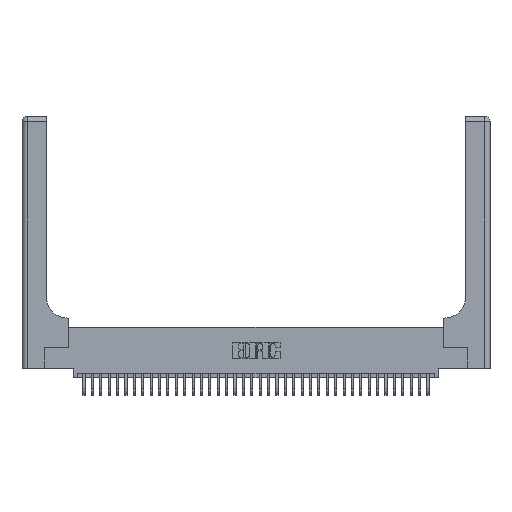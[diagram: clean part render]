
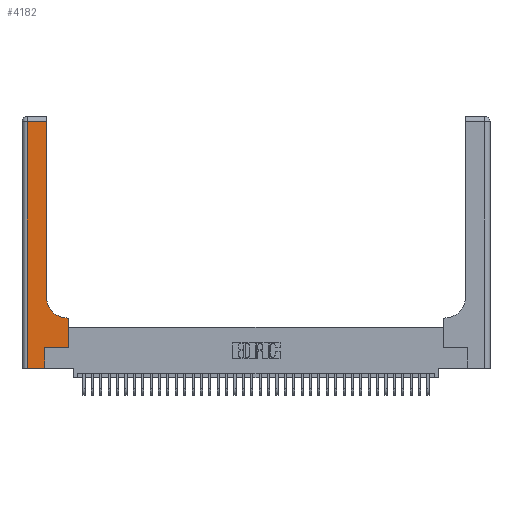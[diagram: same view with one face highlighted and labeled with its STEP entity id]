
A CAD part, top view. The second image highlights one B-rep face of the part: STEP entity #4182.
In plain terms, the highlighted planar face has unit normal (0, 0, 1).
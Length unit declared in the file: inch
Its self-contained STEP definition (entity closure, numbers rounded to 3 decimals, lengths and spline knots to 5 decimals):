
#35 = EDGE_CURVE ( 'NONE', #37936, #5996, #28060, .T. ) ;
#514 = CARTESIAN_POINT ( 'NONE',  ( 0., 0., 0.37 ) ) ;
#1296 = EDGE_CURVE ( 'NONE', #23925, #3361, #37200, .T. ) ;
#1332 = ORIENTED_EDGE ( 'NONE', *, *, #4130, .T. ) ;
#1995 = VECTOR ( 'NONE', #19127, 39.37008 ) ;
#2058 = EDGE_CURVE ( 'NONE', #7646, #23925, #10102, .T. ) ;
#2326 = FACE_OUTER_BOUND ( 'NONE', #29178, .T. ) ;
#3023 = DIRECTION ( 'NONE',  ( 0., 1., 0. ) ) ;
#3274 = LINE ( 'NONE', #15315, #38043 ) ;
#3361 = VERTEX_POINT ( 'NONE', #17592 ) ;
#4130 = EDGE_CURVE ( 'NONE', #7385, #7646, #3274, .T. ) ;
#4182 = ADVANCED_FACE ( 'NONE', ( #2326 ), #16324, .F. ) ;
#4996 = DIRECTION ( 'NONE',  ( 0., 0., -1. ) ) ;
#5067 = DIRECTION ( 'NONE',  ( 0., 1., 0. ) ) ;
#5996 = VERTEX_POINT ( 'NONE', #13791 ) ;
#6104 = AXIS2_PLACEMENT_3D ( 'NONE', #37421, #21985, #6981 ) ;
#6981 = DIRECTION ( 'NONE',  ( 1., 0., 0. ) ) ;
#6991 = CARTESIAN_POINT ( 'NONE',  ( 0.2915, 0.6, 0.37 ) ) ;
#7378 = VERTEX_POINT ( 'NONE', #14151 ) ;
#7385 = VERTEX_POINT ( 'NONE', #11038 ) ;
#7646 = VERTEX_POINT ( 'NONE', #20036 ) ;
#7947 = CARTESIAN_POINT ( 'NONE',  ( 0., 3., 0.37 ) ) ;
#9427 = DIRECTION ( 'NONE',  ( 1., 0., 0. ) ) ;
#10094 = VECTOR ( 'NONE', #13402, 39.37008 ) ;
#10102 = LINE ( 'NONE', #6991, #19773 ) ;
#10522 = VECTOR ( 'NONE', #5067, 39.37008 ) ;
#11038 = CARTESIAN_POINT ( 'NONE',  ( 0.5585, 0.25, 0.37 ) ) ;
#11072 = DIRECTION ( 'NONE',  ( -1., 0., 0. ) ) ;
#11276 = CARTESIAN_POINT ( 'NONE',  ( 0.269, 0., 0.37 ) ) ;
#11614 = VECTOR ( 'NONE', #38617, 39.37008 ) ;
#12543 = LINE ( 'NONE', #32020, #10094 ) ;
#12682 = ORIENTED_EDGE ( 'NONE', *, *, #39432, .T. ) ;
#12975 = ORIENTED_EDGE ( 'NONE', *, *, #1296, .T. ) ;
#13402 = DIRECTION ( 'NONE',  ( 0., -1., 0. ) ) ;
#13417 = ORIENTED_EDGE ( 'NONE', *, *, #23449, .T. ) ;
#13592 = CARTESIAN_POINT ( 'NONE',  ( 0.2915, 2.94, 0.37 ) ) ;
#13791 = CARTESIAN_POINT ( 'NONE',  ( 0.06, 2.94, 0.37 ) ) ;
#13945 = CARTESIAN_POINT ( 'NONE',  ( 0., 2.94, 0.37 ) ) ;
#14151 = CARTESIAN_POINT ( 'NONE',  ( 0.06, 0., 0.37 ) ) ;
#14584 = CARTESIAN_POINT ( 'NONE',  ( 0.269, 0., 0.37 ) ) ;
#15315 = CARTESIAN_POINT ( 'NONE',  ( 0.5585, 0.25, 0.37 ) ) ;
#15416 = LINE ( 'NONE', #11276, #10522 ) ;
#16324 = PLANE ( 'NONE',  #31753 ) ;
#17295 = DIRECTION ( 'NONE',  ( -1., 0., 0. ) ) ;
#17592 = CARTESIAN_POINT ( 'NONE',  ( 0.2915, 0.85, 0.37 ) ) ;
#19127 = DIRECTION ( 'NONE',  ( 1., 0., 0. ) ) ;
#19310 = CARTESIAN_POINT ( 'NONE',  ( 0.269, 0.25, 0.37 ) ) ;
#19773 = VECTOR ( 'NONE', #37948, 39.37008 ) ;
#19787 = LINE ( 'NONE', #35820, #11614 ) ;
#20036 = CARTESIAN_POINT ( 'NONE',  ( 0.5585, 0.6, 0.37 ) ) ;
#20267 = LINE ( 'NONE', #514, #1995 ) ;
#21985 = DIRECTION ( 'NONE',  ( 0., 0., -1. ) ) ;
#22276 = CARTESIAN_POINT ( 'NONE',  ( 0.5415, 0.6, 0.37 ) ) ;
#23449 = EDGE_CURVE ( 'NONE', #28666, #23914, #15416, .T. ) ;
#23914 = VERTEX_POINT ( 'NONE', #19310 ) ;
#23925 = VERTEX_POINT ( 'NONE', #22276 ) ;
#26183 = ORIENTED_EDGE ( 'NONE', *, *, #34802, .T. ) ;
#28013 = CARTESIAN_POINT ( 'NONE',  ( 0.269, 0.25, 0.37 ) ) ;
#28060 = LINE ( 'NONE', #13945, #34375 ) ;
#28533 = ORIENTED_EDGE ( 'NONE', *, *, #2058, .T. ) ;
#28666 = VERTEX_POINT ( 'NONE', #14584 ) ;
#29178 = EDGE_LOOP ( 'NONE', ( #12682, #32243, #31343, #26183, #13417, #29841, #1332, #28533, #12975 ) ) ;
#29841 = ORIENTED_EDGE ( 'NONE', *, *, #37742, .T. ) ;
#31343 = ORIENTED_EDGE ( 'NONE', *, *, #32334, .T. ) ;
#31753 = AXIS2_PLACEMENT_3D ( 'NONE', #7947, #4996, #11072 ) ;
#32020 = CARTESIAN_POINT ( 'NONE',  ( 0.06, 3., 0.37 ) ) ;
#32243 = ORIENTED_EDGE ( 'NONE', *, *, #35, .T. ) ;
#32334 = EDGE_CURVE ( 'NONE', #5996, #7378, #12543, .T. ) ;
#33449 = VECTOR ( 'NONE', #9427, 39.37008 ) ;
#34375 = VECTOR ( 'NONE', #17295, 39.37008 ) ;
#34802 = EDGE_CURVE ( 'NONE', #7378, #28666, #20267, .T. ) ;
#35820 = CARTESIAN_POINT ( 'NONE',  ( 0.2915, 3., 0.37 ) ) ;
#37200 = CIRCLE ( 'NONE', #6104, 0.25 ) ;
#37421 = CARTESIAN_POINT ( 'NONE',  ( 0.5415, 0.85, 0.37 ) ) ;
#37742 = EDGE_CURVE ( 'NONE', #23914, #7385, #39737, .T. ) ;
#37936 = VERTEX_POINT ( 'NONE', #13592 ) ;
#37948 = DIRECTION ( 'NONE',  ( -1., 0., 0. ) ) ;
#38043 = VECTOR ( 'NONE', #3023, 39.37008 ) ;
#38617 = DIRECTION ( 'NONE',  ( 0., 1., 0. ) ) ;
#39432 = EDGE_CURVE ( 'NONE', #3361, #37936, #19787, .T. ) ;
#39737 = LINE ( 'NONE', #28013, #33449 ) ;
